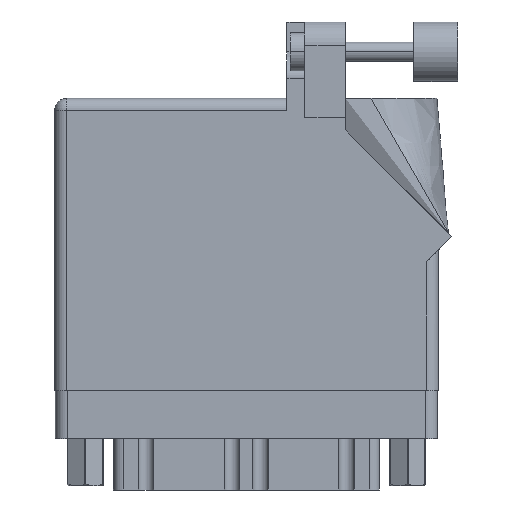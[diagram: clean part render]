
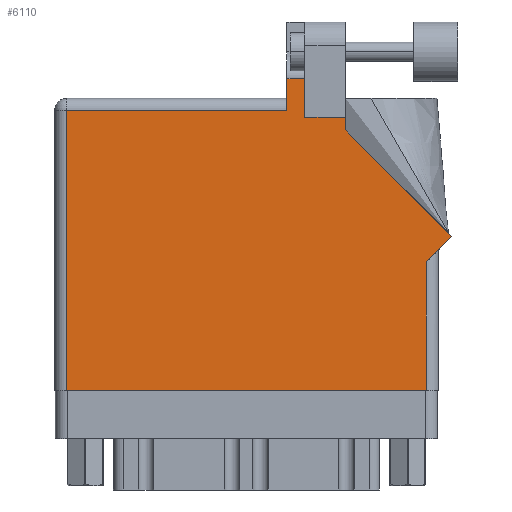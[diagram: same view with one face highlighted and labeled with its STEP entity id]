
A CAD part, front view. The second image highlights one B-rep face of the part: STEP entity #6110.
In plain terms, the highlighted face is planar.
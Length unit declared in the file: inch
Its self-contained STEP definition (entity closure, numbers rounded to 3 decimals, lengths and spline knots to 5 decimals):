
#321 = CARTESIAN_POINT ( 'NONE',  ( 0.062, 0., 0. ) ) ;
#877 = CARTESIAN_POINT ( 'NONE',  ( 1.64177, 1.6315, 0. ) ) ;
#1159 = DIRECTION ( 'NONE',  ( 0., 1., 0. ) ) ;
#2186 = VERTEX_POINT ( 'NONE', #34749 ) ;
#2228 = VECTOR ( 'NONE', #34326, 39.37008 ) ;
#2570 = VERTEX_POINT ( 'NONE', #22343 ) ;
#2642 = EDGE_CURVE ( 'NONE', #2570, #5558, #15535, .T. ) ;
#2674 = EDGE_CURVE ( 'NONE', #39931, #35671, #41959, .T. ) ;
#3382 = CARTESIAN_POINT ( 'NONE',  ( 1.311, 1.43, 0. ) ) ;
#3463 = LINE ( 'NONE', #14349, #35317 ) ;
#4269 = LINE ( 'NONE', #877, #2228 ) ;
#4548 = LINE ( 'NONE', #34843, #18588 ) ;
#5558 = VERTEX_POINT ( 'NONE', #23353 ) ;
#6110 = ADVANCED_FACE ( 'NONE', ( #46478 ), #21031, .F. ) ;
#6234 = DIRECTION ( 'NONE',  ( 0.707, 0.707, 0. ) ) ;
#6318 = VERTEX_POINT ( 'NONE', #23066 ) ;
#7091 = DIRECTION ( 'NONE',  ( 1., 0., 0. ) ) ;
#8070 = VERTEX_POINT ( 'NONE', #17215 ) ;
#8143 = CARTESIAN_POINT ( 'NONE',  ( 2.08071, 0.80771, 0. ) ) ;
#8572 = VECTOR ( 'NONE', #6234, 39.37008 ) ;
#9115 = EDGE_CURVE ( 'NONE', #29456, #39931, #3463, .T. ) ;
#9860 = DIRECTION ( 'NONE',  ( 0., 0., -1. ) ) ;
#10068 = EDGE_CURVE ( 'NONE', #5558, #29456, #40530, .T. ) ;
#11456 = VECTOR ( 'NONE', #22130, 39.37008 ) ;
#12074 = LINE ( 'NONE', #13026, #32165 ) ;
#12401 = VECTOR ( 'NONE', #29159, 39.37008 ) ;
#12611 = EDGE_CURVE ( 'NONE', #31230, #21313, #12074, .T. ) ;
#12625 = CARTESIAN_POINT ( 'NONE',  ( 0., 1.468, 0. ) ) ;
#13026 = CARTESIAN_POINT ( 'NONE',  ( 1.524, 1.43, 0. ) ) ;
#13059 = ORIENTED_EDGE ( 'NONE', *, *, #2642, .T. ) ;
#13550 = ORIENTED_EDGE ( 'NONE', *, *, #9115, .T. ) ;
#13628 = ORIENTED_EDGE ( 'NONE', *, *, #12611, .T. ) ;
#14349 = CARTESIAN_POINT ( 'NONE',  ( 0., 0., 0. ) ) ;
#14796 = VECTOR ( 'NONE', #44942, 39.37008 ) ;
#15535 = LINE ( 'NONE', #12625, #46254 ) ;
#16012 = DIRECTION ( 'NONE',  ( 0., 1., 0. ) ) ;
#16202 = EDGE_LOOP ( 'NONE', ( #36878, #36418, #28403, #13059, #47609, #13550, #24496, #45208, #21811, #18027, #13628 ) ) ;
#16251 = DIRECTION ( 'NONE',  ( -1., 0., 0. ) ) ;
#17215 = CARTESIAN_POINT ( 'NONE',  ( 1.217, 1.6315, 0. ) ) ;
#18027 = ORIENTED_EDGE ( 'NONE', *, *, #45610, .T. ) ;
#18588 = VECTOR ( 'NONE', #1159, 39.37008 ) ;
#20519 = EDGE_CURVE ( 'NONE', #2186, #8070, #4269, .T. ) ;
#21031 = PLANE ( 'NONE',  #34917 ) ;
#21313 = VERTEX_POINT ( 'NONE', #3382 ) ;
#21811 = ORIENTED_EDGE ( 'NONE', *, *, #23935, .T. ) ;
#22130 = DIRECTION ( 'NONE',  ( 0., 1., 0. ) ) ;
#22343 = CARTESIAN_POINT ( 'NONE',  ( 1.217, 1.468, 0. ) ) ;
#22874 = LINE ( 'NONE', #37178, #14796 ) ;
#23051 = VECTOR ( 'NONE', #16012, 39.37008 ) ;
#23066 = CARTESIAN_POINT ( 'NONE',  ( 2.08071, 0.80771, 0. ) ) ;
#23353 = CARTESIAN_POINT ( 'NONE',  ( 0.062, 1.468, 0. ) ) ;
#23935 = EDGE_CURVE ( 'NONE', #6318, #38352, #41353, .T. ) ;
#24496 = ORIENTED_EDGE ( 'NONE', *, *, #2674, .T. ) ;
#25033 = LINE ( 'NONE', #36176, #11456 ) ;
#25116 = EDGE_CURVE ( 'NONE', #35671, #6318, #43311, .T. ) ;
#25635 = EDGE_CURVE ( 'NONE', #8070, #2570, #22874, .T. ) ;
#27846 = CARTESIAN_POINT ( 'NONE',  ( 0.062, 0., 0. ) ) ;
#28331 = CARTESIAN_POINT ( 'NONE',  ( 1.948, 0., 0. ) ) ;
#28403 = ORIENTED_EDGE ( 'NONE', *, *, #25635, .T. ) ;
#28681 = CARTESIAN_POINT ( 'NONE',  ( 1.524, 1.36442, 0. ) ) ;
#29159 = DIRECTION ( 'NONE',  ( 0., -1., 0. ) ) ;
#29456 = VERTEX_POINT ( 'NONE', #27846 ) ;
#30220 = CARTESIAN_POINT ( 'NONE',  ( 1.948, 0.675, 0. ) ) ;
#31230 = VERTEX_POINT ( 'NONE', #40290 ) ;
#31925 = CARTESIAN_POINT ( 'NONE',  ( 2.01, 0.737, 0. ) ) ;
#32165 = VECTOR ( 'NONE', #38949, 39.37008 ) ;
#34326 = DIRECTION ( 'NONE',  ( -1., 0., 0. ) ) ;
#34749 = CARTESIAN_POINT ( 'NONE',  ( 1.311, 1.6315, 0. ) ) ;
#34843 = CARTESIAN_POINT ( 'NONE',  ( 1.311, 1.43, 0. ) ) ;
#34917 = AXIS2_PLACEMENT_3D ( 'NONE', #35811, #9860, #46957 ) ;
#34931 = CARTESIAN_POINT ( 'NONE',  ( 1.948, 0.737, 0. ) ) ;
#35317 = VECTOR ( 'NONE', #7091, 39.37008 ) ;
#35671 = VERTEX_POINT ( 'NONE', #30220 ) ;
#35811 = CARTESIAN_POINT ( 'NONE',  ( 0., 1.53, 0. ) ) ;
#36176 = CARTESIAN_POINT ( 'NONE',  ( 1.524, 1.36442, 0. ) ) ;
#36418 = ORIENTED_EDGE ( 'NONE', *, *, #20519, .T. ) ;
#36878 = ORIENTED_EDGE ( 'NONE', *, *, #40277, .T. ) ;
#37178 = CARTESIAN_POINT ( 'NONE',  ( 1.217, 1.53, 0. ) ) ;
#38352 = VERTEX_POINT ( 'NONE', #28681 ) ;
#38949 = DIRECTION ( 'NONE',  ( -1., 0., 0. ) ) ;
#39931 = VERTEX_POINT ( 'NONE', #28331 ) ;
#40277 = EDGE_CURVE ( 'NONE', #21313, #2186, #4548, .T. ) ;
#40290 = CARTESIAN_POINT ( 'NONE',  ( 1.524, 1.43, 0. ) ) ;
#40530 = LINE ( 'NONE', #321, #12401 ) ;
#41353 = LINE ( 'NONE', #8143, #42659 ) ;
#41959 = LINE ( 'NONE', #34931, #23051 ) ;
#42659 = VECTOR ( 'NONE', #43266, 39.37008 ) ;
#43266 = DIRECTION ( 'NONE',  ( -0.707, 0.707, 0. ) ) ;
#43311 = LINE ( 'NONE', #31925, #8572 ) ;
#44942 = DIRECTION ( 'NONE',  ( 0., -1., 0. ) ) ;
#45208 = ORIENTED_EDGE ( 'NONE', *, *, #25116, .T. ) ;
#45610 = EDGE_CURVE ( 'NONE', #38352, #31230, #25033, .T. ) ;
#46254 = VECTOR ( 'NONE', #16251, 39.37008 ) ;
#46478 = FACE_OUTER_BOUND ( 'NONE', #16202, .T. ) ;
#46957 = DIRECTION ( 'NONE',  ( -1., 0., 0. ) ) ;
#47609 = ORIENTED_EDGE ( 'NONE', *, *, #10068, .T. ) ;
